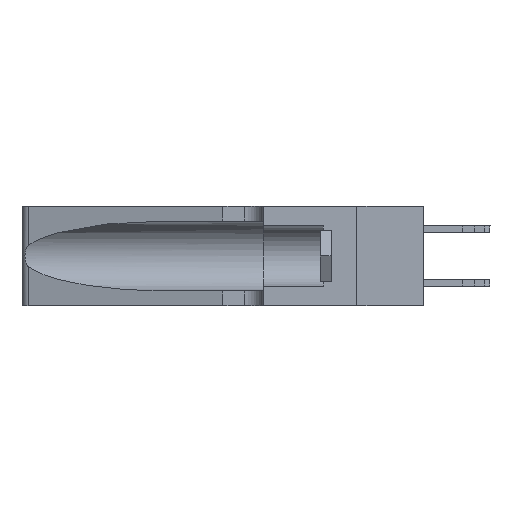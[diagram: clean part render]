
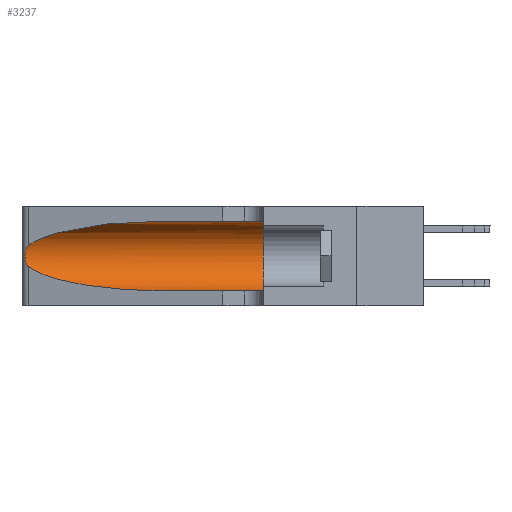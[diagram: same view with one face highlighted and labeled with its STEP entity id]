
A CAD part, left-side view. The second image highlights one B-rep face of the part: STEP entity #3237.
In plain terms, the highlighted cylindrical face has radius 3.308 mm (diameter 6.617 mm), a partial arc.
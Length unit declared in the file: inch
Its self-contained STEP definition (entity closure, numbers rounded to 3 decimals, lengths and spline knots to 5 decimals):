
#301 = DIRECTION ( 'NONE',  ( 0., 0., 1. ) ) ;
#408 = VERTEX_POINT ( 'NONE', #12329 ) ;
#848 = CARTESIAN_POINT ( 'NONE',  ( 0.25639, 1.23186, 0.15144 ) ) ;
#973 = CARTESIAN_POINT ( 'NONE',  ( 0.26075, 1.23896, 0.178 ) ) ;
#1097 = CARTESIAN_POINT ( 'NONE',  ( 0.25789, 1.23486, 0.15765 ) ) ;
#1724 = VECTOR ( 'NONE', #13505, 39.37008 ) ;
#1768 = FACE_OUTER_BOUND ( 'NONE', #13632, .T. ) ;
#2178 = CARTESIAN_POINT ( 'NONE',  ( 0.25487, 1.22718, 0.14631 ) ) ;
#2261 = EDGE_CURVE ( 'NONE', #4677, #10568, #7409, .T. ) ;
#2321 = CARTESIAN_POINT ( 'NONE',  ( 0.1305, 0.72297, 0.05475 ) ) ;
#2536 = CARTESIAN_POINT ( 'NONE',  ( 0.1305, 1.61858, 0.185 ) ) ;
#3237 = ADVANCED_FACE ( 'NONE', ( #1768 ), #14697, .F. ) ;
#3304 = CARTESIAN_POINT ( 'NONE',  ( 0.1305, 0.35, 0.185 ) ) ;
#3852 = CARTESIAN_POINT ( 'NONE',  ( 0.26017, 1.23833, 0.17102 ) ) ;
#3919 = EDGE_CURVE ( 'NONE', #8527, #10896, #15969, .T. ) ;
#4168 = AXIS2_PLACEMENT_3D ( 'NONE', #3304, #14447, #301 ) ;
#4677 = VERTEX_POINT ( 'NONE', #7670 ) ;
#4696 = VECTOR ( 'NONE', #10904, 39.37008 ) ;
#5067 = CARTESIAN_POINT ( 'NONE',  ( 0.1305, 0.72297, 0.31525 ) ) ;
#5139 = CARTESIAN_POINT ( 'NONE',  ( 0.25555, 1.22994, 0.2215 ) ) ;
#5140 = CARTESIAN_POINT ( 'NONE',  ( 0.18966, 0.96281, 0.05475 ) ) ;
#5149 = CARTESIAN_POINT ( 'NONE',  ( 0.2373, 1.15595, 0.28018 ) ) ;
#5519 = EDGE_CURVE ( 'NONE', #10896, #408, #13913, .T. ) ;
#6011 = LINE ( 'NONE', #15082, #4696 ) ;
#6493 = CARTESIAN_POINT ( 'NONE',  ( 0.25487, 1.22718, 0.14631 ) ) ;
#6527 = EDGE_CURVE ( 'NONE', #10568, #16627, #15857, .T. ) ;
#6550 = CARTESIAN_POINT ( 'NONE',  ( 0.25787, 1.23484, 0.2124 ) ) ;
#6611 = CARTESIAN_POINT ( 'NONE',  ( 0.25639, 1.23184, 0.21858 ) ) ;
#7243 = ORIENTED_EDGE ( 'NONE', *, *, #2261, .T. ) ;
#7308 = DIRECTION ( 'NONE',  ( 0., 0., -1. ) ) ;
#7409 = B_SPLINE_CURVE_WITH_KNOTS ( 'NONE', 3,
 ( #10699, #5139, #6611, #6550, #13692, #9481, #13566, #973, #3852, #9232, #1097, #848, #10638, #7906 ),
 .UNSPECIFIED., .F., .F.,
 ( 4, 2, 2, 2, 2, 2, 4 ),
 ( 0., 0.00027, 0.00053, 0.00107, 0.0016, 0.00187, 0.00214 ),
 .UNSPECIFIED. ) ;
#7670 = CARTESIAN_POINT ( 'NONE',  ( 0.25487, 1.22718, 0.22369 ) ) ;
#7906 = CARTESIAN_POINT ( 'NONE',  ( 0.25487, 1.22718, 0.14631 ) ) ;
#8243 = CARTESIAN_POINT ( 'NONE',  ( 0.1305, 0.35, 0.31525 ) ) ;
#8527 = VERTEX_POINT ( 'NONE', #5067 ) ;
#8543 =( BOUNDED_CURVE ( )  B_SPLINE_CURVE ( 3, ( #16252, #9185, #5149, #14951 ),
 .UNSPECIFIED., .F., .T. ) 
 B_SPLINE_CURVE_WITH_KNOTS ( ( 4, 4 ),
 ( 1.5708, 2.84003 ),
 .UNSPECIFIED. ) 
 CURVE ( )  GEOMETRIC_REPRESENTATION_ITEM ( )  RATIONAL_B_SPLINE_CURVE ( ( 1., 0.87, 0.87, 1. ) ) 
 REPRESENTATION_ITEM ( '' )  );
#9185 = CARTESIAN_POINT ( 'NONE',  ( 0.18966, 0.96281, 0.31525 ) ) ;
#9232 = CARTESIAN_POINT ( 'NONE',  ( 0.25856, 1.23593, 0.16098 ) ) ;
#9481 = CARTESIAN_POINT ( 'NONE',  ( 0.26018, 1.23835, 0.19895 ) ) ;
#10568 = VERTEX_POINT ( 'NONE', #2178 ) ;
#10638 = CARTESIAN_POINT ( 'NONE',  ( 0.25555, 1.22993, 0.14849 ) ) ;
#10699 = CARTESIAN_POINT ( 'NONE',  ( 0.25487, 1.22718, 0.22369 ) ) ;
#10896 = VERTEX_POINT ( 'NONE', #8243 ) ;
#10904 = DIRECTION ( 'NONE',  ( 0., -1., 0. ) ) ;
#11527 = ORIENTED_EDGE ( 'NONE', *, *, #6527, .T. ) ;
#12063 = CARTESIAN_POINT ( 'NONE',  ( 0.1305, 1.61858, 0.31525 ) ) ;
#12329 = CARTESIAN_POINT ( 'NONE',  ( 0.1305, 0.35, 0.05475 ) ) ;
#13268 = CARTESIAN_POINT ( 'NONE',  ( 0.1305, 0.72297, 0.05475 ) ) ;
#13505 = DIRECTION ( 'NONE',  ( 0., -1., 0. ) ) ;
#13566 = CARTESIAN_POINT ( 'NONE',  ( 0.26075, 1.23896, 0.19203 ) ) ;
#13632 = EDGE_LOOP ( 'NONE', ( #15252, #7243, #11527, #14184, #17570, #15942 ) ) ;
#13643 = AXIS2_PLACEMENT_3D ( 'NONE', #2536, #14281, #7308 ) ;
#13692 = CARTESIAN_POINT ( 'NONE',  ( 0.25854, 1.2359, 0.20912 ) ) ;
#13913 = CIRCLE ( 'NONE', #4168, 0.13025 ) ;
#14184 = ORIENTED_EDGE ( 'NONE', *, *, #16079, .T. ) ;
#14281 = DIRECTION ( 'NONE',  ( 0., -1., 0. ) ) ;
#14447 = DIRECTION ( 'NONE',  ( 0., 1., 0. ) ) ;
#14617 = EDGE_CURVE ( 'NONE', #8527, #4677, #8543, .T. ) ;
#14697 = CYLINDRICAL_SURFACE ( 'NONE', #13643, 0.13025 ) ;
#14939 = CARTESIAN_POINT ( 'NONE',  ( 0.2373, 1.15595, 0.08982 ) ) ;
#14951 = CARTESIAN_POINT ( 'NONE',  ( 0.25487, 1.22718, 0.22369 ) ) ;
#15082 = CARTESIAN_POINT ( 'NONE',  ( 0.1305, 1.61858, 0.05475 ) ) ;
#15252 = ORIENTED_EDGE ( 'NONE', *, *, #14617, .T. ) ;
#15857 =( BOUNDED_CURVE ( )  B_SPLINE_CURVE ( 3, ( #6493, #14939, #5140, #2321 ),
 .UNSPECIFIED., .F., .F. ) 
 B_SPLINE_CURVE_WITH_KNOTS ( ( 4, 4 ),
 ( 3.44316, 4.71239 ),
 .UNSPECIFIED. ) 
 CURVE ( )  GEOMETRIC_REPRESENTATION_ITEM ( )  RATIONAL_B_SPLINE_CURVE ( ( 1., 0.87, 0.87, 1. ) ) 
 REPRESENTATION_ITEM ( '' )  );
#15942 = ORIENTED_EDGE ( 'NONE', *, *, #3919, .F. ) ;
#15969 = LINE ( 'NONE', #12063, #1724 ) ;
#16079 = EDGE_CURVE ( 'NONE', #16627, #408, #6011, .T. ) ;
#16252 = CARTESIAN_POINT ( 'NONE',  ( 0.1305, 0.72297, 0.31525 ) ) ;
#16627 = VERTEX_POINT ( 'NONE', #13268 ) ;
#17570 = ORIENTED_EDGE ( 'NONE', *, *, #5519, .F. ) ;
